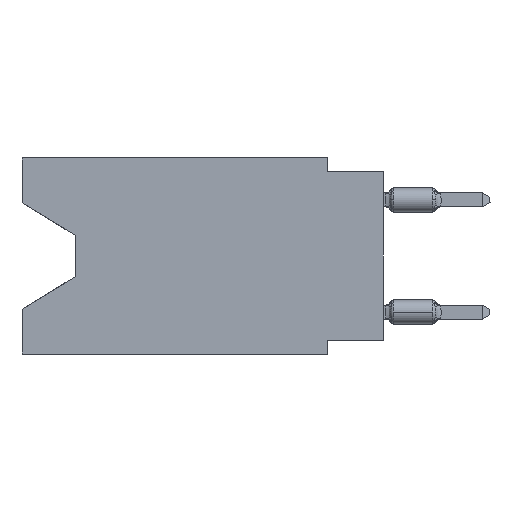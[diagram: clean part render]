
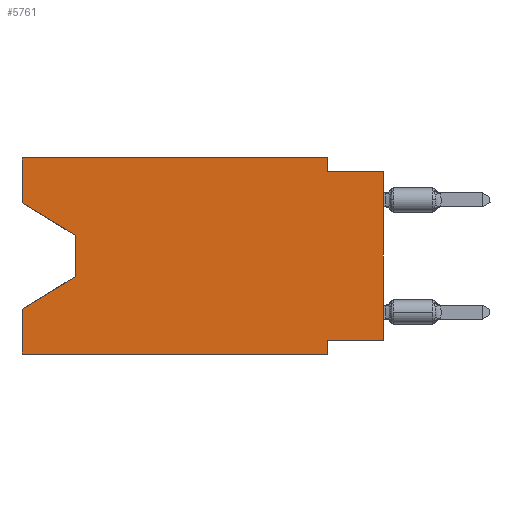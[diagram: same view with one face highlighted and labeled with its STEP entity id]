
A CAD part, left-side view. The second image highlights one B-rep face of the part: STEP entity #5761.
In plain terms, the highlighted planar face has unit normal (-1, 0, 0).
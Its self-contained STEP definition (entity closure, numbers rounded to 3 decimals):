
#362 = VECTOR ( 'NONE', #35750, 1000. ) ;
#725 = VERTEX_POINT ( 'NONE', #18720 ) ;
#831 = EDGE_CURVE ( 'NONE', #30074, #14726, #16434, .T. ) ;
#1142 = CARTESIAN_POINT ( 'NONE',  ( 0., 16.383, -8.89 ) ) ;
#1150 = CARTESIAN_POINT ( 'NONE',  ( 0., 0., -8.255 ) ) ;
#1334 = LINE ( 'NONE', #1150, #4489 ) ;
#1507 = VERTEX_POINT ( 'NONE', #27140 ) ;
#1804 = DIRECTION ( 'NONE',  ( 0., 0., -1. ) ) ;
#2699 = CARTESIAN_POINT ( 'NONE',  ( 0., 2.54, -8.255 ) ) ;
#4028 = EDGE_CURVE ( 'NONE', #725, #29079, #25333, .T. ) ;
#4489 = VECTOR ( 'NONE', #35342, 1000. ) ;
#4805 = CARTESIAN_POINT ( 'NONE',  ( 0., 16.383, 0. ) ) ;
#4933 = LINE ( 'NONE', #13650, #22087 ) ;
#5544 = VERTEX_POINT ( 'NONE', #35188 ) ;
#5595 = DIRECTION ( 'NONE',  ( 0., 0.855, -0.519 ) ) ;
#5761 = ADVANCED_FACE ( 'NONE', ( #22213 ), #33737, .F. ) ;
#6147 = DIRECTION ( 'NONE',  ( 0., 0., -1. ) ) ;
#6676 = EDGE_CURVE ( 'NONE', #14551, #5544, #34215, .T. ) ;
#6844 = VECTOR ( 'NONE', #21925, 1000. ) ;
#7852 = CARTESIAN_POINT ( 'NONE',  ( 0., 16.383, 0. ) ) ;
#8512 = VERTEX_POINT ( 'NONE', #2699 ) ;
#8724 = DIRECTION ( 'NONE',  ( 0., 0., 1. ) ) ;
#8833 = ORIENTED_EDGE ( 'NONE', *, *, #24836, .F. ) ;
#10196 = DIRECTION ( 'NONE',  ( 0., 0., -1. ) ) ;
#10881 = LINE ( 'NONE', #30541, #21071 ) ;
#10963 = DIRECTION ( 'NONE',  ( 0., 0., 1. ) ) ;
#10981 = DIRECTION ( 'NONE',  ( 0., -1., 0. ) ) ;
#11011 = ORIENTED_EDGE ( 'NONE', *, *, #33430, .T. ) ;
#11052 = EDGE_CURVE ( 'NONE', #5544, #25189, #34092, .T. ) ;
#12338 = AXIS2_PLACEMENT_3D ( 'NONE', #7852, #30909, #10196 ) ;
#13096 = CARTESIAN_POINT ( 'NONE',  ( 0., 16.383, -2.038 ) ) ;
#13255 = CARTESIAN_POINT ( 'NONE',  ( 0., 0., -0.635 ) ) ;
#13619 = CARTESIAN_POINT ( 'NONE',  ( 0., 0., 0. ) ) ;
#13650 = CARTESIAN_POINT ( 'NONE',  ( 0., 16.383, 0. ) ) ;
#13809 = CARTESIAN_POINT ( 'NONE',  ( 0., 16.383, 0. ) ) ;
#14551 = VERTEX_POINT ( 'NONE', #33710 ) ;
#14726 = VERTEX_POINT ( 'NONE', #34650 ) ;
#14890 = CARTESIAN_POINT ( 'NONE',  ( 0., 2.54, -8.89 ) ) ;
#14910 = ORIENTED_EDGE ( 'NONE', *, *, #24596, .T. ) ;
#14913 = ORIENTED_EDGE ( 'NONE', *, *, #36264, .F. ) ;
#15891 = ORIENTED_EDGE ( 'NONE', *, *, #831, .T. ) ;
#15944 = ORIENTED_EDGE ( 'NONE', *, *, #4028, .F. ) ;
#16356 = DIRECTION ( 'NONE',  ( 0., -1., 0. ) ) ;
#16434 = LINE ( 'NONE', #19262, #27636 ) ;
#16541 = EDGE_CURVE ( 'NONE', #29462, #8512, #1334, .T. ) ;
#18276 = ORIENTED_EDGE ( 'NONE', *, *, #11052, .F. ) ;
#18720 = CARTESIAN_POINT ( 'NONE',  ( 0., 2.54, -0.635 ) ) ;
#18770 = LINE ( 'NONE', #13096, #362 ) ;
#18779 = ORIENTED_EDGE ( 'NONE', *, *, #6676, .F. ) ;
#19256 = VERTEX_POINT ( 'NONE', #34809 ) ;
#19262 = CARTESIAN_POINT ( 'NONE',  ( 0., 16.383, -8.89 ) ) ;
#19535 = CARTESIAN_POINT ( 'NONE',  ( 0., 13.97, -5.385 ) ) ;
#19975 = LINE ( 'NONE', #31497, #21899 ) ;
#20337 = LINE ( 'NONE', #25994, #22136 ) ;
#20548 = LINE ( 'NONE', #14890, #21163 ) ;
#21071 = VECTOR ( 'NONE', #1804, 1000. ) ;
#21096 = CARTESIAN_POINT ( 'NONE',  ( 0., 2.54, 0. ) ) ;
#21163 = VECTOR ( 'NONE', #23566, 1000. ) ;
#21856 = CARTESIAN_POINT ( 'NONE',  ( 0., 0., -0.635 ) ) ;
#21899 = VECTOR ( 'NONE', #5595, 1000. ) ;
#21925 = DIRECTION ( 'NONE',  ( 0., 0., 1. ) ) ;
#22087 = VECTOR ( 'NONE', #8724, 1000. ) ;
#22136 = VECTOR ( 'NONE', #6147, 1000. ) ;
#22213 = FACE_OUTER_BOUND ( 'NONE', #27476, .T. ) ;
#22843 = ORIENTED_EDGE ( 'NONE', *, *, #26108, .T. ) ;
#23070 = VERTEX_POINT ( 'NONE', #19535 ) ;
#23566 = DIRECTION ( 'NONE',  ( 0., 0., -1. ) ) ;
#23840 = VECTOR ( 'NONE', #10981, 1000. ) ;
#24596 = EDGE_CURVE ( 'NONE', #14551, #1507, #18770, .T. ) ;
#24836 = EDGE_CURVE ( 'NONE', #30074, #19256, #4933, .T. ) ;
#25189 = VERTEX_POINT ( 'NONE', #21096 ) ;
#25333 = LINE ( 'NONE', #13255, #23840 ) ;
#25994 = CARTESIAN_POINT ( 'NONE',  ( 0., 2.54, 0. ) ) ;
#26108 = EDGE_CURVE ( 'NONE', #29462, #29079, #36826, .T. ) ;
#26540 = EDGE_CURVE ( 'NONE', #23070, #19256, #19975, .T. ) ;
#27140 = CARTESIAN_POINT ( 'NONE',  ( 0., 13.97, -3.505 ) ) ;
#27476 = EDGE_LOOP ( 'NONE', ( #14910, #11011, #28540, #8833, #15891, #14913, #37232, #22843, #15944, #32527, #18276, #18779 ) ) ;
#27636 = VECTOR ( 'NONE', #28334, 1000. ) ;
#28334 = DIRECTION ( 'NONE',  ( 0., -1., 0. ) ) ;
#28540 = ORIENTED_EDGE ( 'NONE', *, *, #26540, .T. ) ;
#29079 = VERTEX_POINT ( 'NONE', #21856 ) ;
#29134 = VECTOR ( 'NONE', #10963, 1000. ) ;
#29462 = VERTEX_POINT ( 'NONE', #30917 ) ;
#30074 = VERTEX_POINT ( 'NONE', #1142 ) ;
#30541 = CARTESIAN_POINT ( 'NONE',  ( 0., 13.97, -3.505 ) ) ;
#30838 = EDGE_CURVE ( 'NONE', #25189, #725, #20337, .T. ) ;
#30909 = DIRECTION ( 'NONE',  ( 1., 0., 0. ) ) ;
#30917 = CARTESIAN_POINT ( 'NONE',  ( 0., 0., -8.255 ) ) ;
#31497 = CARTESIAN_POINT ( 'NONE',  ( 0., 13.97, -5.385 ) ) ;
#32527 = ORIENTED_EDGE ( 'NONE', *, *, #30838, .F. ) ;
#33430 = EDGE_CURVE ( 'NONE', #1507, #23070, #10881, .T. ) ;
#33498 = VECTOR ( 'NONE', #16356, 1000. ) ;
#33710 = CARTESIAN_POINT ( 'NONE',  ( 0., 16.383, -2.038 ) ) ;
#33737 = PLANE ( 'NONE',  #12338 ) ;
#34092 = LINE ( 'NONE', #4805, #33498 ) ;
#34215 = LINE ( 'NONE', #13809, #6844 ) ;
#34650 = CARTESIAN_POINT ( 'NONE',  ( 0., 2.54, -8.89 ) ) ;
#34809 = CARTESIAN_POINT ( 'NONE',  ( 0., 16.383, -6.852 ) ) ;
#35188 = CARTESIAN_POINT ( 'NONE',  ( 0., 16.383, 0. ) ) ;
#35342 = DIRECTION ( 'NONE',  ( 0., 1., 0. ) ) ;
#35750 = DIRECTION ( 'NONE',  ( 0., -0.855, -0.519 ) ) ;
#36264 = EDGE_CURVE ( 'NONE', #8512, #14726, #20548, .T. ) ;
#36826 = LINE ( 'NONE', #13619, #29134 ) ;
#37232 = ORIENTED_EDGE ( 'NONE', *, *, #16541, .F. ) ;
